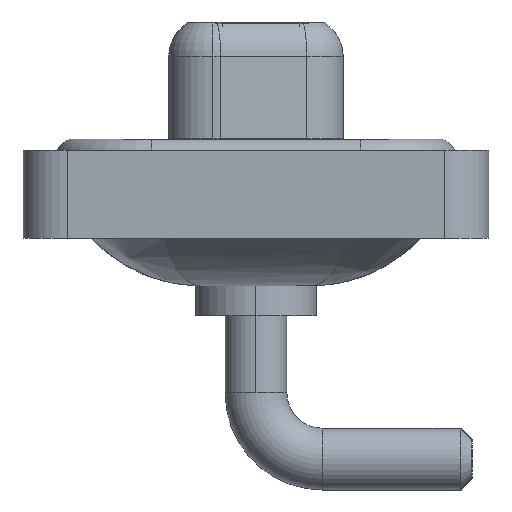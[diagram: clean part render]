
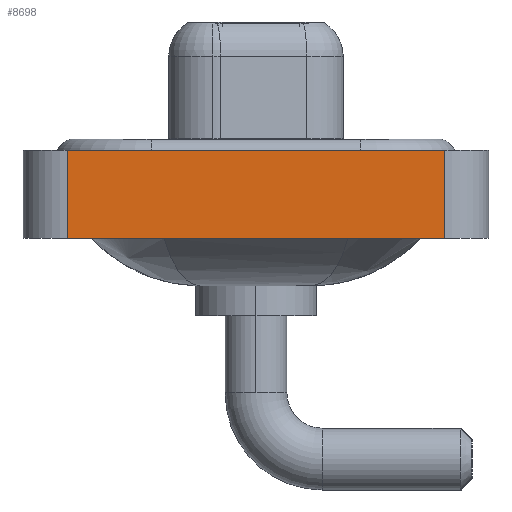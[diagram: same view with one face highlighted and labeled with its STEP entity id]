
A CAD part, left-side view. The second image highlights one B-rep face of the part: STEP entity #8698.
In plain terms, the highlighted planar face has unit normal (-1, 0, 0).
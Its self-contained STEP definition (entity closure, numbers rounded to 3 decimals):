
#249 = VECTOR ( 'NONE', #968, 1000. ) ;
#502 = VERTEX_POINT ( 'NONE', #794 ) ;
#794 = CARTESIAN_POINT ( 'NONE',  ( -7.3, 8.55, 0.4 ) ) ;
#968 = DIRECTION ( 'NONE',  ( 0., -1., 0. ) ) ;
#1120 = VECTOR ( 'NONE', #12279, 1000. ) ;
#1404 = CARTESIAN_POINT ( 'NONE',  ( -7.3, -8.55, -3.6 ) ) ;
#1956 = EDGE_CURVE ( 'NONE', #4024, #10878, #14210, .T. ) ;
#2956 = ORIENTED_EDGE ( 'NONE', *, *, #1956, .T. ) ;
#3177 = CARTESIAN_POINT ( 'NONE',  ( -7.3, -8.55, 0.4 ) ) ;
#3266 = ORIENTED_EDGE ( 'NONE', *, *, #12941, .F. ) ;
#3711 = VECTOR ( 'NONE', #6977, 1000. ) ;
#4024 = VERTEX_POINT ( 'NONE', #11458 ) ;
#4035 = LINE ( 'NONE', #1404, #1120 ) ;
#5705 = DIRECTION ( 'NONE',  ( -1., 0., 0. ) ) ;
#6119 = EDGE_CURVE ( 'NONE', #502, #6486, #15208, .T. ) ;
#6203 = CARTESIAN_POINT ( 'NONE',  ( -7.3, -8.55, -3.6 ) ) ;
#6246 = CARTESIAN_POINT ( 'NONE',  ( -7.3, -8.55, -3.6 ) ) ;
#6486 = VERTEX_POINT ( 'NONE', #9976 ) ;
#6877 = CARTESIAN_POINT ( 'NONE',  ( -7.3, 8.55, -3.6 ) ) ;
#6977 = DIRECTION ( 'NONE',  ( 0., -1., 0. ) ) ;
#7052 = LINE ( 'NONE', #6877, #12523 ) ;
#7692 = ORIENTED_EDGE ( 'NONE', *, *, #8579, .T. ) ;
#8579 = EDGE_CURVE ( 'NONE', #10878, #6486, #4035, .T. ) ;
#8698 = ADVANCED_FACE ( 'NONE', ( #12530 ), #10054, .T. ) ;
#9702 = CARTESIAN_POINT ( 'NONE',  ( -7.3, -8.55, -3.6 ) ) ;
#9976 = CARTESIAN_POINT ( 'NONE',  ( -7.3, -8.55, 0.4 ) ) ;
#10054 = PLANE ( 'NONE',  #14090 ) ;
#10878 = VERTEX_POINT ( 'NONE', #6203 ) ;
#11458 = CARTESIAN_POINT ( 'NONE',  ( -7.3, 8.55, -3.6 ) ) ;
#12279 = DIRECTION ( 'NONE',  ( 0., 0., 1. ) ) ;
#12294 = DIRECTION ( 'NONE',  ( 0., 0., 1. ) ) ;
#12523 = VECTOR ( 'NONE', #12294, 1000. ) ;
#12530 = FACE_OUTER_BOUND ( 'NONE', #15673, .T. ) ;
#12941 = EDGE_CURVE ( 'NONE', #4024, #502, #7052, .T. ) ;
#13073 = ORIENTED_EDGE ( 'NONE', *, *, #6119, .F. ) ;
#13851 = DIRECTION ( 'NONE',  ( 0., 0., 1. ) ) ;
#14090 = AXIS2_PLACEMENT_3D ( 'NONE', #9702, #5705, #13851 ) ;
#14210 = LINE ( 'NONE', #6246, #249 ) ;
#15208 = LINE ( 'NONE', #3177, #3711 ) ;
#15673 = EDGE_LOOP ( 'NONE', ( #7692, #13073, #3266, #2956 ) ) ;
